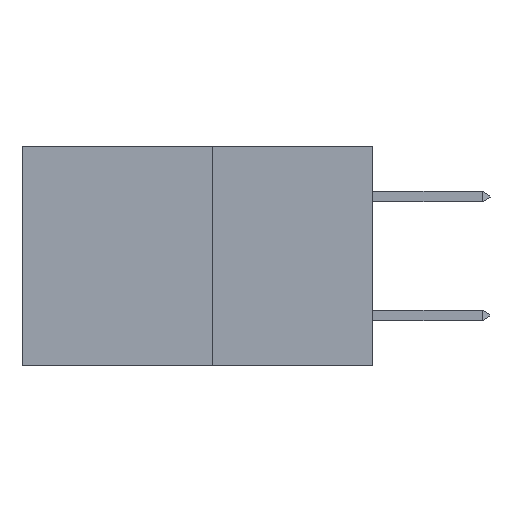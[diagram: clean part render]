
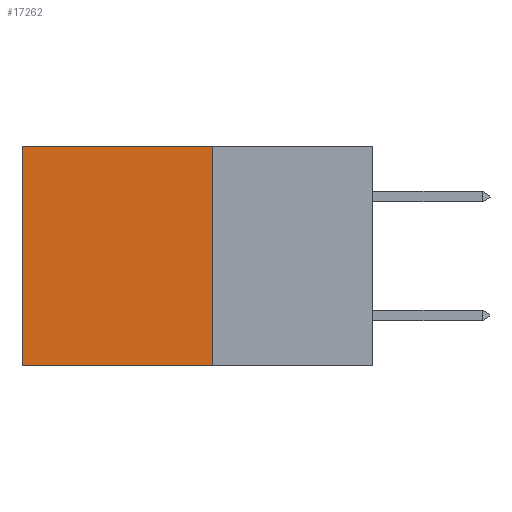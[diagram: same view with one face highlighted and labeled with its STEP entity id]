
A CAD part, left-side view. The second image highlights one B-rep face of the part: STEP entity #17262.
In plain terms, the highlighted planar face has unit normal (-1, 0, 0).
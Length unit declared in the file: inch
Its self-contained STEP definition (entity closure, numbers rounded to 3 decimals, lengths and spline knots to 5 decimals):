
#401 = DIRECTION ( 'NONE',  ( 0., 0., -1. ) ) ;
#1751 = CARTESIAN_POINT ( 'NONE',  ( 0.277, 0.27, -0.37 ) ) ;
#2511 = CARTESIAN_POINT ( 'NONE',  ( 0.277, 0.59, 0. ) ) ;
#2878 = DIRECTION ( 'NONE',  ( 0., 1., 0. ) ) ;
#3528 = EDGE_CURVE ( 'NONE', #14594, #9072, #11401, .T. ) ;
#3980 = LINE ( 'NONE', #16230, #11873 ) ;
#4126 = EDGE_CURVE ( 'NONE', #9072, #14112, #5532, .T. ) ;
#4166 = CARTESIAN_POINT ( 'NONE',  ( 0.277, 0.59, -0.37 ) ) ;
#4436 = FACE_OUTER_BOUND ( 'NONE', #13070, .T. ) ;
#4895 = ORIENTED_EDGE ( 'NONE', *, *, #17736, .T. ) ;
#5532 = LINE ( 'NONE', #15912, #8979 ) ;
#6111 = DIRECTION ( 'NONE',  ( 0., 0., -1. ) ) ;
#6162 = VECTOR ( 'NONE', #401, 39.37008 ) ;
#6253 = CARTESIAN_POINT ( 'NONE',  ( 0.277, 0.59, -0.37 ) ) ;
#6354 = EDGE_CURVE ( 'NONE', #17003, #14112, #10845, .T. ) ;
#6735 = CARTESIAN_POINT ( 'NONE',  ( 0.277, 0.27, -0.37 ) ) ;
#8351 = CARTESIAN_POINT ( 'NONE',  ( 0.277, 0.27, -0.37 ) ) ;
#8979 = VECTOR ( 'NONE', #18797, 39.37008 ) ;
#9072 = VERTEX_POINT ( 'NONE', #6735 ) ;
#10845 = LINE ( 'NONE', #6253, #6162 ) ;
#11401 = LINE ( 'NONE', #8351, #18562 ) ;
#11873 = VECTOR ( 'NONE', #2878, 39.37008 ) ;
#12113 = PLANE ( 'NONE',  #18659 ) ;
#13070 = EDGE_LOOP ( 'NONE', ( #13905, #13176, #13883, #4895 ) ) ;
#13176 = ORIENTED_EDGE ( 'NONE', *, *, #4126, .F. ) ;
#13835 = DIRECTION ( 'NONE',  ( 0., 0., -1. ) ) ;
#13883 = ORIENTED_EDGE ( 'NONE', *, *, #3528, .F. ) ;
#13905 = ORIENTED_EDGE ( 'NONE', *, *, #6354, .T. ) ;
#14112 = VERTEX_POINT ( 'NONE', #4166 ) ;
#14371 = CARTESIAN_POINT ( 'NONE',  ( 0.277, 0.27, 0. ) ) ;
#14594 = VERTEX_POINT ( 'NONE', #14371 ) ;
#15078 = DIRECTION ( 'NONE',  ( 1., 0., 0. ) ) ;
#15912 = CARTESIAN_POINT ( 'NONE',  ( 0.277, 0.27, -0.37 ) ) ;
#16230 = CARTESIAN_POINT ( 'NONE',  ( 0.277, 0.27, 0. ) ) ;
#17003 = VERTEX_POINT ( 'NONE', #2511 ) ;
#17262 = ADVANCED_FACE ( 'NONE', ( #4436 ), #12113, .F. ) ;
#17736 = EDGE_CURVE ( 'NONE', #14594, #17003, #3980, .T. ) ;
#18562 = VECTOR ( 'NONE', #13835, 39.37008 ) ;
#18659 = AXIS2_PLACEMENT_3D ( 'NONE', #1751, #15078, #6111 ) ;
#18797 = DIRECTION ( 'NONE',  ( 0., 1., 0. ) ) ;
